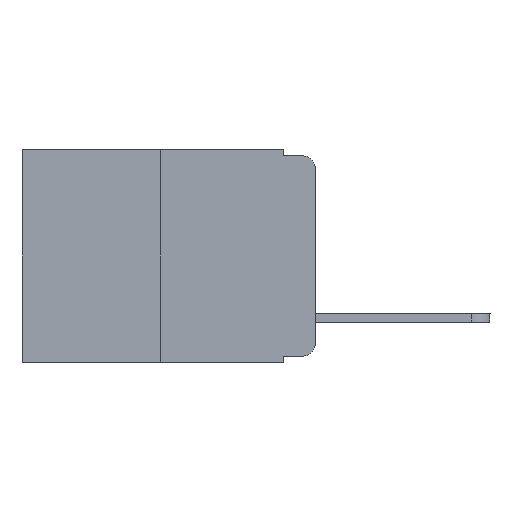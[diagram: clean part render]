
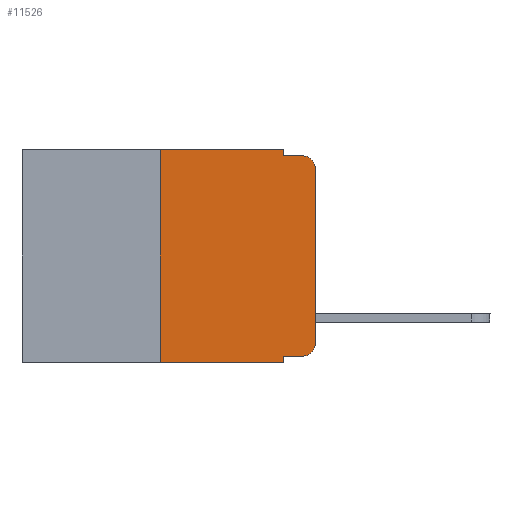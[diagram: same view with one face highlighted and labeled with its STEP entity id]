
A CAD part, left-side view. The second image highlights one B-rep face of the part: STEP entity #11526.
In plain terms, the highlighted planar face has unit normal (-1, 0, 0).
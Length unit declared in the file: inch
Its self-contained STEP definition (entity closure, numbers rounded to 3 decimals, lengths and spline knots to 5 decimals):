
#16 = ORIENTED_EDGE ( 'NONE', *, *, #9127, .F. ) ;
#17 = EDGE_CURVE ( 'NONE', #6172, #9390, #2761, .T. ) ;
#23 = LINE ( 'NONE', #4788, #6627 ) ;
#106 = DIRECTION ( 'NONE',  ( 0., 0., -1. ) ) ;
#474 = AXIS2_PLACEMENT_3D ( 'NONE', #12264, #12186, #13295 ) ;
#545 = DIRECTION ( 'NONE',  ( -1., 0., 0. ) ) ;
#768 = CARTESIAN_POINT ( 'NONE',  ( 0., 0.25, 0. ) ) ;
#1292 = EDGE_CURVE ( 'NONE', #9390, #6958, #13502, .T. ) ;
#1377 = CARTESIAN_POINT ( 'NONE',  ( 0., 0., -0.313 ) ) ;
#1418 = ORIENTED_EDGE ( 'NONE', *, *, #7141, .F. ) ;
#1423 = CARTESIAN_POINT ( 'NONE',  ( 0., 0.051, -0.333 ) ) ;
#1578 = VECTOR ( 'NONE', #5336, 39.37008 ) ;
#1579 = CARTESIAN_POINT ( 'NONE',  ( 0., 0.051, -0.333 ) ) ;
#1745 = CARTESIAN_POINT ( 'NONE',  ( 0., 0.473, 0. ) ) ;
#1898 = ORIENTED_EDGE ( 'NONE', *, *, #10335, .F. ) ;
#2352 = EDGE_CURVE ( 'NONE', #8913, #6172, #7703, .T. ) ;
#2584 = LINE ( 'NONE', #10945, #10773 ) ;
#2608 = CARTESIAN_POINT ( 'NONE',  ( 0., 0.25, 0. ) ) ;
#2646 = LINE ( 'NONE', #1423, #5784 ) ;
#2761 = LINE ( 'NONE', #9814, #8810 ) ;
#3077 = AXIS2_PLACEMENT_3D ( 'NONE', #6850, #5589, #13887 ) ;
#3539 = VERTEX_POINT ( 'NONE', #8213 ) ;
#3588 = CARTESIAN_POINT ( 'NONE',  ( 0., 0.02, -0.01 ) ) ;
#4485 = FACE_OUTER_BOUND ( 'NONE', #8808, .T. ) ;
#4487 = ORIENTED_EDGE ( 'NONE', *, *, #17, .T. ) ;
#4741 = CARTESIAN_POINT ( 'NONE',  ( 0., 0.051, 0. ) ) ;
#4788 = CARTESIAN_POINT ( 'NONE',  ( 0., 0.051, 0. ) ) ;
#5013 = DIRECTION ( 'NONE',  ( 0., -1., 0. ) ) ;
#5299 = CARTESIAN_POINT ( 'NONE',  ( 0., 0.02, -0.03 ) ) ;
#5336 = DIRECTION ( 'NONE',  ( 0., -1., 0. ) ) ;
#5589 = DIRECTION ( 'NONE',  ( 1., 0., 0. ) ) ;
#5629 = EDGE_CURVE ( 'NONE', #13514, #11163, #14206, .T. ) ;
#5704 = VERTEX_POINT ( 'NONE', #13267 ) ;
#5784 = VECTOR ( 'NONE', #7424, 39.37008 ) ;
#6042 = EDGE_CURVE ( 'NONE', #3539, #11163, #11760, .T. ) ;
#6172 = VERTEX_POINT ( 'NONE', #1377 ) ;
#6581 = EDGE_CURVE ( 'NONE', #13604, #6958, #2584, .T. ) ;
#6627 = VECTOR ( 'NONE', #106, 39.37008 ) ;
#6709 = ORIENTED_EDGE ( 'NONE', *, *, #13234, .T. ) ;
#6739 = VECTOR ( 'NONE', #6927, 39.37008 ) ;
#6850 = CARTESIAN_POINT ( 'NONE',  ( 0., 0.473, 0. ) ) ;
#6890 = CARTESIAN_POINT ( 'NONE',  ( 0., 0., -0.03 ) ) ;
#6927 = DIRECTION ( 'NONE',  ( 0., -1., 0. ) ) ;
#6958 = VERTEX_POINT ( 'NONE', #3588 ) ;
#7141 = EDGE_CURVE ( 'NONE', #3539, #7463, #12621, .T. ) ;
#7424 = DIRECTION ( 'NONE',  ( 0., -1., 0. ) ) ;
#7463 = VERTEX_POINT ( 'NONE', #2608 ) ;
#7476 = ORIENTED_EDGE ( 'NONE', *, *, #5629, .F. ) ;
#7703 = CIRCLE ( 'NONE', #474, 0.02 ) ;
#7948 = DIRECTION ( 'NONE',  ( 0., 0., -1. ) ) ;
#8213 = CARTESIAN_POINT ( 'NONE',  ( 0., 0.25, -0.343 ) ) ;
#8808 = EDGE_LOOP ( 'NONE', ( #4487, #13732, #12383, #1898, #16, #1418, #13200, #7476, #6709, #14680 ) ) ;
#8810 = VECTOR ( 'NONE', #11057, 39.37008 ) ;
#8913 = VERTEX_POINT ( 'NONE', #10206 ) ;
#9127 = EDGE_CURVE ( 'NONE', #7463, #5704, #14798, .T. ) ;
#9390 = VERTEX_POINT ( 'NONE', #6890 ) ;
#9814 = CARTESIAN_POINT ( 'NONE',  ( 0., 0., 0. ) ) ;
#10206 = CARTESIAN_POINT ( 'NONE',  ( 0., 0.02, -0.333 ) ) ;
#10335 = EDGE_CURVE ( 'NONE', #5704, #13604, #23, .T. ) ;
#10403 = CARTESIAN_POINT ( 'NONE',  ( 0., 0.051, -0.01 ) ) ;
#10773 = VECTOR ( 'NONE', #5013, 39.37008 ) ;
#10945 = CARTESIAN_POINT ( 'NONE',  ( 0., 0.051, -0.01 ) ) ;
#11057 = DIRECTION ( 'NONE',  ( 0., 0., 1. ) ) ;
#11163 = VERTEX_POINT ( 'NONE', #14055 ) ;
#11526 = ADVANCED_FACE ( 'NONE', ( #4485 ), #11755, .F. ) ;
#11563 = VECTOR ( 'NONE', #13896, 39.37008 ) ;
#11754 = AXIS2_PLACEMENT_3D ( 'NONE', #5299, #545, #7948 ) ;
#11755 = PLANE ( 'NONE',  #3077 ) ;
#11760 = LINE ( 'NONE', #15275, #6739 ) ;
#12186 = DIRECTION ( 'NONE',  ( -1., 0., 0. ) ) ;
#12264 = CARTESIAN_POINT ( 'NONE',  ( 0., 0.02, -0.313 ) ) ;
#12383 = ORIENTED_EDGE ( 'NONE', *, *, #6581, .F. ) ;
#12621 = LINE ( 'NONE', #768, #11563 ) ;
#13200 = ORIENTED_EDGE ( 'NONE', *, *, #6042, .T. ) ;
#13234 = EDGE_CURVE ( 'NONE', #13514, #8913, #2646, .T. ) ;
#13267 = CARTESIAN_POINT ( 'NONE',  ( 0., 0.051, 0. ) ) ;
#13295 = DIRECTION ( 'NONE',  ( 0., 0., -1. ) ) ;
#13502 = CIRCLE ( 'NONE', #11754, 0.02 ) ;
#13514 = VERTEX_POINT ( 'NONE', #1579 ) ;
#13604 = VERTEX_POINT ( 'NONE', #10403 ) ;
#13732 = ORIENTED_EDGE ( 'NONE', *, *, #1292, .T. ) ;
#13887 = DIRECTION ( 'NONE',  ( 0., 0., -1. ) ) ;
#13896 = DIRECTION ( 'NONE',  ( 0., 0., 1. ) ) ;
#13986 = DIRECTION ( 'NONE',  ( 0., 0., -1. ) ) ;
#14055 = CARTESIAN_POINT ( 'NONE',  ( 0., 0.051, -0.343 ) ) ;
#14206 = LINE ( 'NONE', #4741, #15056 ) ;
#14680 = ORIENTED_EDGE ( 'NONE', *, *, #2352, .T. ) ;
#14798 = LINE ( 'NONE', #1745, #1578 ) ;
#15056 = VECTOR ( 'NONE', #13986, 39.37008 ) ;
#15275 = CARTESIAN_POINT ( 'NONE',  ( 0., 0.473, -0.343 ) ) ;
